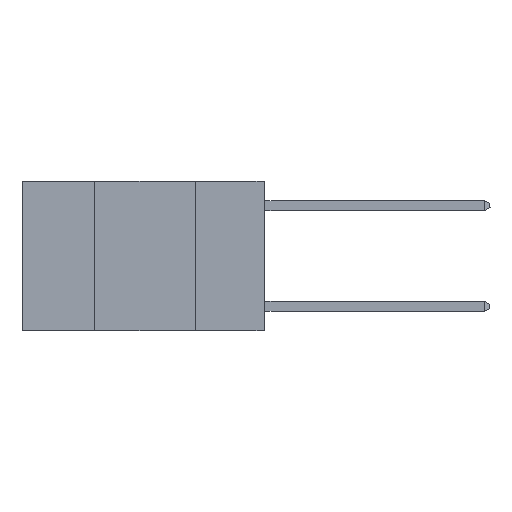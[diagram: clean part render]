
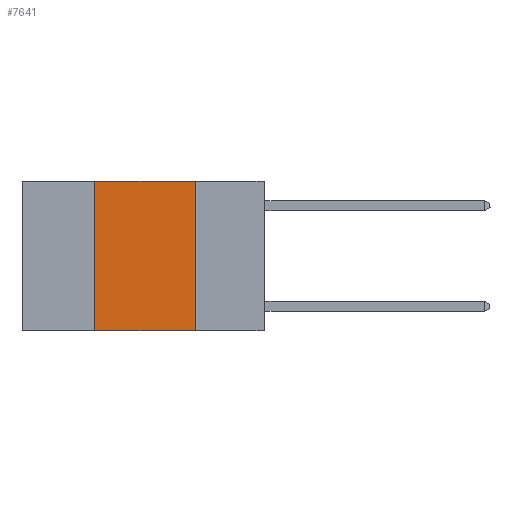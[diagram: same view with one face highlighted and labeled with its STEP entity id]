
A CAD part, left-side view. The second image highlights one B-rep face of the part: STEP entity #7641.
In plain terms, the highlighted planar face has unit normal (-1, 0, 0).
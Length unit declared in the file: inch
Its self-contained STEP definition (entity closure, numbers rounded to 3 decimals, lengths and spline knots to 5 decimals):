
#71 = DIRECTION ( 'NONE',  ( 0., 0., -1. ) ) ;
#498 = ORIENTED_EDGE ( 'NONE', *, *, #17200, .F. ) ;
#1383 = LINE ( 'NONE', #15133, #9337 ) ;
#3232 = CARTESIAN_POINT ( 'NONE',  ( 0., 0.42, -0.37 ) ) ;
#3306 = CARTESIAN_POINT ( 'NONE',  ( 0., 0.42, 0. ) ) ;
#3439 = VERTEX_POINT ( 'NONE', #3306 ) ;
#3806 = VERTEX_POINT ( 'NONE', #18597 ) ;
#4458 = VECTOR ( 'NONE', #7827, 39.37008 ) ;
#4870 = CARTESIAN_POINT ( 'NONE',  ( 0., 0.6, 0. ) ) ;
#5056 = CARTESIAN_POINT ( 'NONE',  ( 0., 0.6, -0.37 ) ) ;
#5257 = LINE ( 'NONE', #5056, #8937 ) ;
#5374 = AXIS2_PLACEMENT_3D ( 'NONE', #4870, #9608, #71 ) ;
#6299 = CARTESIAN_POINT ( 'NONE',  ( 0., 0.6, 0. ) ) ;
#7641 = ADVANCED_FACE ( 'NONE', ( #10210 ), #19034, .F. ) ;
#7827 = DIRECTION ( 'NONE',  ( 0., 0., 1. ) ) ;
#8633 = LINE ( 'NONE', #18839, #4458 ) ;
#8709 = VERTEX_POINT ( 'NONE', #19891 ) ;
#8937 = VECTOR ( 'NONE', #14507, 39.37008 ) ;
#8964 = ORIENTED_EDGE ( 'NONE', *, *, #17464, .F. ) ;
#9337 = VECTOR ( 'NONE', #13613, 39.37008 ) ;
#9608 = DIRECTION ( 'NONE',  ( 1., 0., 0. ) ) ;
#10210 = FACE_OUTER_BOUND ( 'NONE', #13113, .T. ) ;
#13113 = EDGE_LOOP ( 'NONE', ( #498, #8964, #13659, #17816 ) ) ;
#13613 = DIRECTION ( 'NONE',  ( 0., 0., -1. ) ) ;
#13659 = ORIENTED_EDGE ( 'NONE', *, *, #16168, .F. ) ;
#13776 = LINE ( 'NONE', #6299, #17439 ) ;
#14507 = DIRECTION ( 'NONE',  ( 0., -1., 0. ) ) ;
#15114 = EDGE_CURVE ( 'NONE', #17516, #3806, #5257, .T. ) ;
#15133 = CARTESIAN_POINT ( 'NONE',  ( 0., 0.17, 0. ) ) ;
#16168 = EDGE_CURVE ( 'NONE', #17516, #3439, #8633, .T. ) ;
#17200 = EDGE_CURVE ( 'NONE', #8709, #3806, #1383, .T. ) ;
#17439 = VECTOR ( 'NONE', #18884, 39.37008 ) ;
#17464 = EDGE_CURVE ( 'NONE', #3439, #8709, #13776, .T. ) ;
#17516 = VERTEX_POINT ( 'NONE', #3232 ) ;
#17816 = ORIENTED_EDGE ( 'NONE', *, *, #15114, .T. ) ;
#18597 = CARTESIAN_POINT ( 'NONE',  ( 0., 0.17, -0.37 ) ) ;
#18839 = CARTESIAN_POINT ( 'NONE',  ( 0., 0.42, 0. ) ) ;
#18884 = DIRECTION ( 'NONE',  ( 0., -1., 0. ) ) ;
#19034 = PLANE ( 'NONE',  #5374 ) ;
#19891 = CARTESIAN_POINT ( 'NONE',  ( 0., 0.17, 0. ) ) ;
